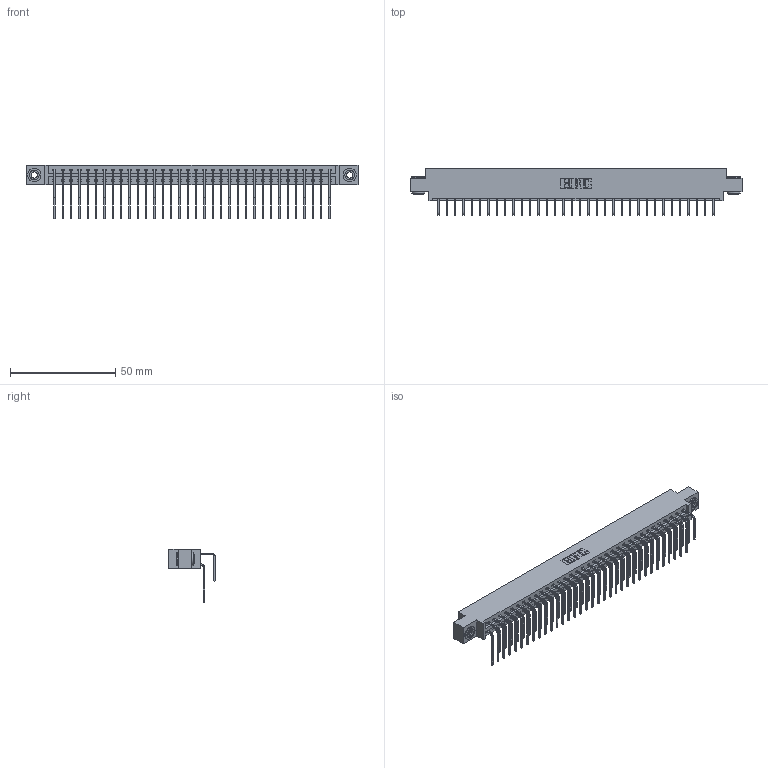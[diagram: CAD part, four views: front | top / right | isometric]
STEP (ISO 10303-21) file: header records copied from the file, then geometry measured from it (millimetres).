
FILE_DESCRIPTION (( 'STEP AP203' ), '1' );
FILE_NAME ('337-068-558-803.STEP', '2019-10-12T02:39:01', ( '' ), ( '' ), 'SwSTEP 2.0', 'SolidWorks 2016', '' );
FILE_SCHEMA (( 'CONFIG_CONTROL_DESIGN' ));
Length unit declared in the file: inch
Products named in the file (5): 345-292-001_558 559 Tail - 1; 337-068-558-803; 345-250-002_345-250-002-102; 337 Part_0.170 Offset - 0.156 Dia-TH; 345-292-001_558 Tail - 2
Assembly tree (71 placements, depth 2):
  337-068-558-803
    337 Part_0.170 Offset - 0.156 Dia-TH
    345-292-001_558 559 Tail - 1  x34
    345-292-001_558 Tail - 2  x34
    345-250-002_345-250-002-102  x2
Bounding box: 157.73 x 22.17 x 25.53 mm (x, y, z)
Volume: 16810.9 mm3; surface area: 21229 mm2
Topology: 71 solids, 71 shells, 3964 faces, 11755 edges, 7742 vertices
Faces by surface type: plane 2804, cylinder 1152, cone 8
Entity records: 29962 total; most frequent: CARTESIAN_POINT 5076, ORIENTED_EDGE 4954, DIRECTION 4347, EDGE_CURVE 2477, VECTOR 2285, LINE 2285, VERTEX_POINT 1646, AXIS2_PLACEMENT_3D 1031
